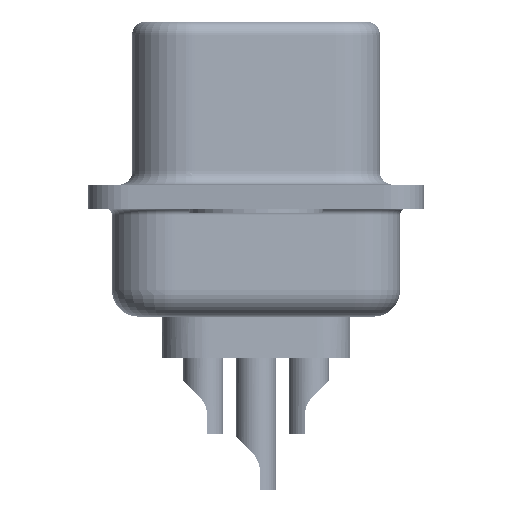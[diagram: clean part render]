
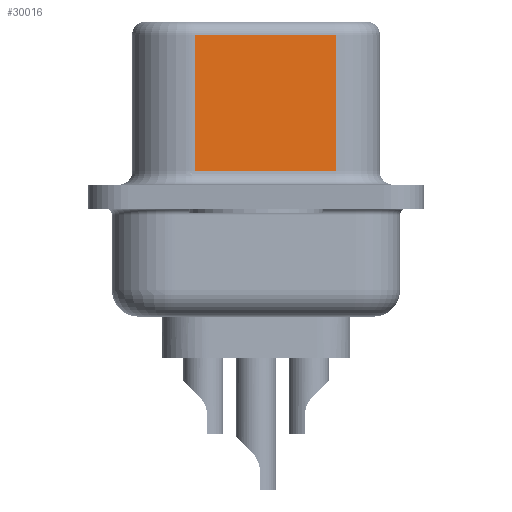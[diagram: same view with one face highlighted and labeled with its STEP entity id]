
A CAD part, left-side view. The second image highlights one B-rep face of the part: STEP entity #30016.
In plain terms, the highlighted planar face has unit normal (-0.985, -0.174, 0).
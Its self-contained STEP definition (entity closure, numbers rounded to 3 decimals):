
#840 = ORIENTED_EDGE ( 'NONE', *, *, #2736, .T. ) ;
#2736 = EDGE_CURVE ( 'NONE', #31033, #22594, #14138, .T. ) ;
#4113 = VERTEX_POINT ( 'NONE', #6006 ) ;
#4623 = EDGE_LOOP ( 'NONE', ( #30216, #840, #22555, #20781 ) ) ;
#4762 = VECTOR ( 'NONE', #29215, 1000. ) ;
#6006 = CARTESIAN_POINT ( 'NONE',  ( 3.62, 2.293, 0.95 ) ) ;
#9621 = CARTESIAN_POINT ( 'NONE',  ( 3.62, 2.293, 6.57 ) ) ;
#9955 = DIRECTION ( 'NONE',  ( 0., 0., -1. ) ) ;
#10342 = CARTESIAN_POINT ( 'NONE',  ( 4.551, -2.987, 6.57 ) ) ;
#11945 = EDGE_CURVE ( 'NONE', #4113, #24144, #26007, .T. ) ;
#12545 = EDGE_CURVE ( 'NONE', #22594, #4113, #22932, .T. ) ;
#13480 = FACE_OUTER_BOUND ( 'NONE', #4623, .T. ) ;
#13966 = DIRECTION ( 'NONE',  ( -0.174, 0.985, 0. ) ) ;
#14138 = LINE ( 'NONE', #22335, #14430 ) ;
#14430 = VECTOR ( 'NONE', #13966, 1000. ) ;
#15686 = DIRECTION ( 'NONE',  ( -0.174, 0.985, 0. ) ) ;
#18320 = CARTESIAN_POINT ( 'NONE',  ( 4.551, -2.987, 0.95 ) ) ;
#18657 = DIRECTION ( 'NONE',  ( 0.174, -0.985, 0. ) ) ;
#20781 = ORIENTED_EDGE ( 'NONE', *, *, #11945, .T. ) ;
#21548 = EDGE_CURVE ( 'NONE', #31033, #24144, #23811, .T. ) ;
#22335 = CARTESIAN_POINT ( 'NONE',  ( 4.551, -2.987, 6.07 ) ) ;
#22555 = ORIENTED_EDGE ( 'NONE', *, *, #12545, .T. ) ;
#22594 = VERTEX_POINT ( 'NONE', #32040 ) ;
#22932 = LINE ( 'NONE', #9621, #31288 ) ;
#23811 = LINE ( 'NONE', #10342, #4762 ) ;
#24144 = VERTEX_POINT ( 'NONE', #31501 ) ;
#24213 = CARTESIAN_POINT ( 'NONE',  ( 4.551, -2.987, 6.57 ) ) ;
#26007 = LINE ( 'NONE', #18320, #32399 ) ;
#27009 = CARTESIAN_POINT ( 'NONE',  ( 4.551, -2.987, 6.07 ) ) ;
#29009 = DIRECTION ( 'NONE',  ( 0.985, 0.174, 0. ) ) ;
#29215 = DIRECTION ( 'NONE',  ( 0., 0., -1. ) ) ;
#30013 = AXIS2_PLACEMENT_3D ( 'NONE', #24213, #29009, #15686 ) ;
#30016 = ADVANCED_FACE ( 'NONE', ( #13480 ), #31889, .F. ) ;
#30216 = ORIENTED_EDGE ( 'NONE', *, *, #21548, .F. ) ;
#31033 = VERTEX_POINT ( 'NONE', #27009 ) ;
#31288 = VECTOR ( 'NONE', #9955, 1000. ) ;
#31501 = CARTESIAN_POINT ( 'NONE',  ( 4.551, -2.987, 0.95 ) ) ;
#31889 = PLANE ( 'NONE',  #30013 ) ;
#32040 = CARTESIAN_POINT ( 'NONE',  ( 3.62, 2.293, 6.07 ) ) ;
#32399 = VECTOR ( 'NONE', #18657, 1000. ) ;
